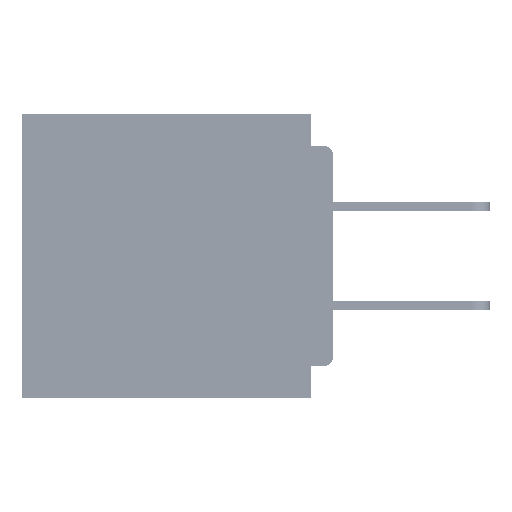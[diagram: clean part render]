
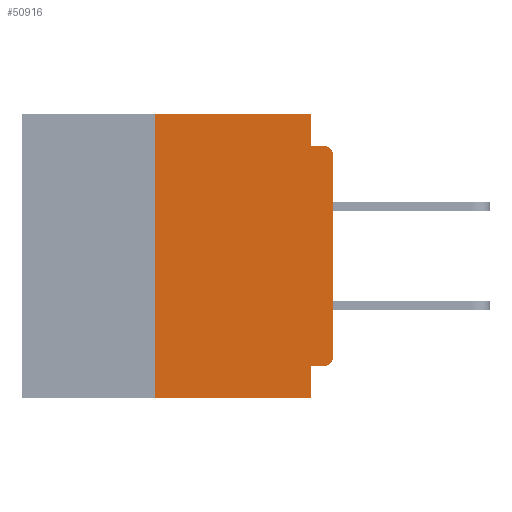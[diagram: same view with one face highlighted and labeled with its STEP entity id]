
A CAD part, left-side view. The second image highlights one B-rep face of the part: STEP entity #50916.
In plain terms, the highlighted planar face has unit normal (-1, 0, 0).
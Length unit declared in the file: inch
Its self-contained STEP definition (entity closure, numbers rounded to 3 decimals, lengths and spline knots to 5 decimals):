
#647 = DIRECTION ( 'NONE',  ( 0., -1., 0. ) ) ;
#1559 = DIRECTION ( 'NONE',  ( 0., 0., -1. ) ) ;
#1679 = PLANE ( 'NONE',  #7480 ) ;
#2778 = ORIENTED_EDGE ( 'NONE', *, *, #57591, .F. ) ;
#6940 = LINE ( 'NONE', #13395, #8562 ) ;
#7446 = VECTOR ( 'NONE', #19968, 39.37008 ) ;
#7480 = AXIS2_PLACEMENT_3D ( 'NONE', #38155, #43377, #12233 ) ;
#8562 = VECTOR ( 'NONE', #49718, 39.37008 ) ;
#8623 = VERTEX_POINT ( 'NONE', #27668 ) ;
#8846 = CARTESIAN_POINT ( 'NONE',  ( 0., 0., -0.06 ) ) ;
#9204 = EDGE_CURVE ( 'NONE', #9481, #49974, #30137, .T. ) ;
#9481 = VERTEX_POINT ( 'NONE', #8846 ) ;
#10203 = CARTESIAN_POINT ( 'NONE',  ( 0., 0.031, 0. ) ) ;
#10541 = DIRECTION ( 'NONE',  ( 0., 0., 1. ) ) ;
#10838 = EDGE_CURVE ( 'NONE', #8623, #47278, #36374, .T. ) ;
#11439 = VECTOR ( 'NONE', #57619, 39.37008 ) ;
#12233 = DIRECTION ( 'NONE',  ( 0., 0., -1. ) ) ;
#13016 = VERTEX_POINT ( 'NONE', #62456 ) ;
#13395 = CARTESIAN_POINT ( 'NONE',  ( 0., 0., 0. ) ) ;
#15094 = ORIENTED_EDGE ( 'NONE', *, *, #59249, .F. ) ;
#15743 = VECTOR ( 'NONE', #647, 39.37008 ) ;
#15825 = ORIENTED_EDGE ( 'NONE', *, *, #29907, .F. ) ;
#15959 = CARTESIAN_POINT ( 'NONE',  ( 0., 0.25, 0. ) ) ;
#18926 = VERTEX_POINT ( 'NONE', #10203 ) ;
#19376 = VERTEX_POINT ( 'NONE', #39946 ) ;
#19968 = DIRECTION ( 'NONE',  ( 0., -1., 0. ) ) ;
#21211 = DIRECTION ( 'NONE',  ( 0., 0., -1. ) ) ;
#21314 = CARTESIAN_POINT ( 'NONE',  ( 0., 0.031, 0. ) ) ;
#21493 = ORIENTED_EDGE ( 'NONE', *, *, #9204, .T. ) ;
#21955 = EDGE_CURVE ( 'NONE', #19376, #49974, #29557, .T. ) ;
#22332 = CARTESIAN_POINT ( 'NONE',  ( 0., 0., -0.34 ) ) ;
#24079 = DIRECTION ( 'NONE',  ( 0., 1., 0. ) ) ;
#24898 = CARTESIAN_POINT ( 'NONE',  ( 0., 0.015, -0.34 ) ) ;
#27642 = CARTESIAN_POINT ( 'NONE',  ( 0., 0.031, -0.4 ) ) ;
#27668 = CARTESIAN_POINT ( 'NONE',  ( 0., 0.015, -0.355 ) ) ;
#28733 = VERTEX_POINT ( 'NONE', #60763 ) ;
#29557 = LINE ( 'NONE', #52560, #15743 ) ;
#29907 = EDGE_CURVE ( 'NONE', #18926, #19376, #40717, .T. ) ;
#30127 = DIRECTION ( 'NONE',  ( 0., 0., -1. ) ) ;
#30137 = CIRCLE ( 'NONE', #57109, 0.015 ) ;
#32836 = DIRECTION ( 'NONE',  ( -1., 0., 0. ) ) ;
#33357 = VERTEX_POINT ( 'NONE', #27642 ) ;
#34227 = CARTESIAN_POINT ( 'NONE',  ( 0., 0.437, 0. ) ) ;
#34654 = LINE ( 'NONE', #55195, #58994 ) ;
#36208 = ORIENTED_EDGE ( 'NONE', *, *, #44222, .T. ) ;
#36374 = CIRCLE ( 'NONE', #58452, 0.015 ) ;
#37654 = LINE ( 'NONE', #57514, #53104 ) ;
#38155 = CARTESIAN_POINT ( 'NONE',  ( 0., 0.437, 0. ) ) ;
#39841 = CARTESIAN_POINT ( 'NONE',  ( 0., 0.015, -0.045 ) ) ;
#39946 = CARTESIAN_POINT ( 'NONE',  ( 0., 0.031, -0.045 ) ) ;
#40717 = LINE ( 'NONE', #21314, #11439 ) ;
#41009 = ORIENTED_EDGE ( 'NONE', *, *, #66148, .F. ) ;
#41163 = FACE_OUTER_BOUND ( 'NONE', #62817, .T. ) ;
#41682 = CARTESIAN_POINT ( 'NONE',  ( 0., 0.25, -0.4 ) ) ;
#41789 = ORIENTED_EDGE ( 'NONE', *, *, #21955, .F. ) ;
#43377 = DIRECTION ( 'NONE',  ( 1., 0., 0. ) ) ;
#44222 = EDGE_CURVE ( 'NONE', #28733, #33357, #62763, .T. ) ;
#44690 = EDGE_CURVE ( 'NONE', #65040, #18926, #59448, .T. ) ;
#45633 = VECTOR ( 'NONE', #65293, 39.37008 ) ;
#47278 = VERTEX_POINT ( 'NONE', #22332 ) ;
#48293 = ORIENTED_EDGE ( 'NONE', *, *, #44690, .F. ) ;
#49718 = DIRECTION ( 'NONE',  ( 0., 0., 1. ) ) ;
#49939 = VECTOR ( 'NONE', #10541, 39.37008 ) ;
#49974 = VERTEX_POINT ( 'NONE', #39841 ) ;
#50916 = ADVANCED_FACE ( 'NONE', ( #41163 ), #1679, .F. ) ;
#52560 = CARTESIAN_POINT ( 'NONE',  ( 0., 0., -0.045 ) ) ;
#53104 = VECTOR ( 'NONE', #21211, 39.37008 ) ;
#55195 = CARTESIAN_POINT ( 'NONE',  ( 0., 0., -0.355 ) ) ;
#56283 = CARTESIAN_POINT ( 'NONE',  ( 0., 0.437, -0.4 ) ) ;
#56392 = ORIENTED_EDGE ( 'NONE', *, *, #65314, .T. ) ;
#57109 = AXIS2_PLACEMENT_3D ( 'NONE', #63884, #32836, #1559 ) ;
#57514 = CARTESIAN_POINT ( 'NONE',  ( 0., 0.031, -0.4 ) ) ;
#57591 = EDGE_CURVE ( 'NONE', #8623, #13016, #34654, .T. ) ;
#57619 = DIRECTION ( 'NONE',  ( 0., 0., -1. ) ) ;
#58452 = AXIS2_PLACEMENT_3D ( 'NONE', #24898, #61206, #30127 ) ;
#58994 = VECTOR ( 'NONE', #24079, 39.37008 ) ;
#59249 = EDGE_CURVE ( 'NONE', #13016, #33357, #37654, .T. ) ;
#59448 = LINE ( 'NONE', #34227, #45633 ) ;
#60763 = CARTESIAN_POINT ( 'NONE',  ( 0., 0.25, -0.4 ) ) ;
#61206 = DIRECTION ( 'NONE',  ( -1., 0., 0. ) ) ;
#62456 = CARTESIAN_POINT ( 'NONE',  ( 0., 0.031, -0.355 ) ) ;
#62763 = LINE ( 'NONE', #56283, #7446 ) ;
#62817 = EDGE_LOOP ( 'NONE', ( #56392, #21493, #41789, #15825, #48293, #41009, #36208, #15094, #2778, #63031 ) ) ;
#63031 = ORIENTED_EDGE ( 'NONE', *, *, #10838, .T. ) ;
#63751 = LINE ( 'NONE', #41682, #49939 ) ;
#63884 = CARTESIAN_POINT ( 'NONE',  ( 0., 0.015, -0.06 ) ) ;
#65040 = VERTEX_POINT ( 'NONE', #15959 ) ;
#65293 = DIRECTION ( 'NONE',  ( 0., -1., 0. ) ) ;
#65314 = EDGE_CURVE ( 'NONE', #47278, #9481, #6940, .T. ) ;
#66148 = EDGE_CURVE ( 'NONE', #28733, #65040, #63751, .T. ) ;
